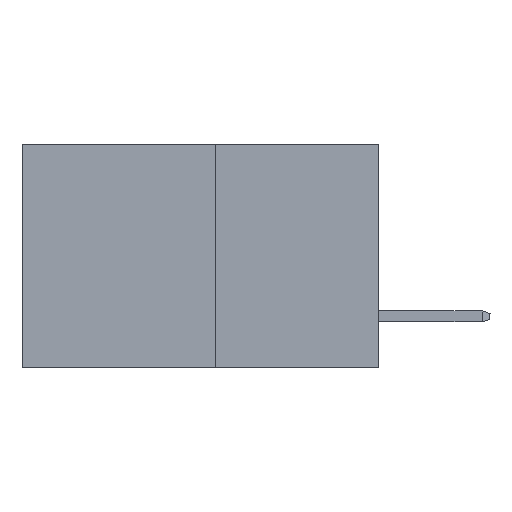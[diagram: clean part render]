
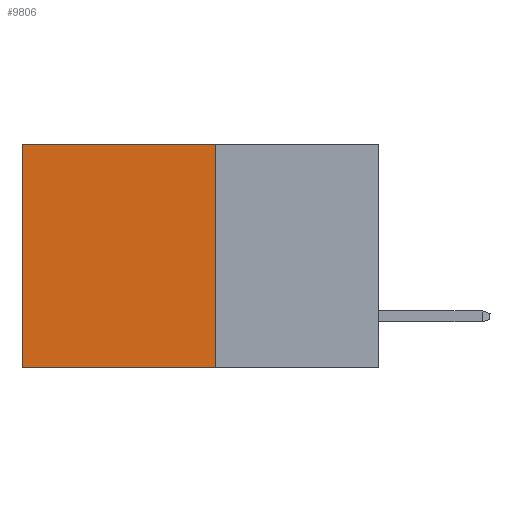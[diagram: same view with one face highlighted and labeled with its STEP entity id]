
A CAD part, left-side view. The second image highlights one B-rep face of the part: STEP entity #9806.
In plain terms, the highlighted planar face has unit normal (-1, 0, 0).
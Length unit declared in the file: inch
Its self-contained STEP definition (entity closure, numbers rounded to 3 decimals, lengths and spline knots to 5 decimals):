
#234 = DIRECTION ( 'NONE',  ( 0., 0., -1. ) ) ;
#895 = LINE ( 'NONE', #8457, #8799 ) ;
#994 = ORIENTED_EDGE ( 'NONE', *, *, #8426, .F. ) ;
#1019 = LINE ( 'NONE', #6784, #7159 ) ;
#1117 = CARTESIAN_POINT ( 'NONE',  ( 0.277, 0.27, -0.37 ) ) ;
#1281 = VERTEX_POINT ( 'NONE', #1923 ) ;
#1366 = VECTOR ( 'NONE', #7724, 39.37008 ) ;
#1373 = DIRECTION ( 'NONE',  ( 1., 0., 0. ) ) ;
#1496 = ORIENTED_EDGE ( 'NONE', *, *, #9750, .T. ) ;
#1528 = VECTOR ( 'NONE', #1953, 39.37008 ) ;
#1857 = VERTEX_POINT ( 'NONE', #4063 ) ;
#1923 = CARTESIAN_POINT ( 'NONE',  ( 0.277, 0.59, 0. ) ) ;
#1953 = DIRECTION ( 'NONE',  ( 0., 1., 0. ) ) ;
#2244 = CARTESIAN_POINT ( 'NONE',  ( 0.277, 0.59, -0.37 ) ) ;
#3518 = LINE ( 'NONE', #9113, #1366 ) ;
#3778 = VERTEX_POINT ( 'NONE', #9079 ) ;
#3937 = LINE ( 'NONE', #1117, #1528 ) ;
#4063 = CARTESIAN_POINT ( 'NONE',  ( 0.277, 0.27, -0.37 ) ) ;
#4882 = EDGE_CURVE ( 'NONE', #1281, #9872, #895, .T. ) ;
#5848 = ORIENTED_EDGE ( 'NONE', *, *, #4882, .T. ) ;
#6466 = EDGE_LOOP ( 'NONE', ( #5848, #8527, #994, #1496 ) ) ;
#6784 = CARTESIAN_POINT ( 'NONE',  ( 0.277, 0.27, -0.37 ) ) ;
#6917 = CARTESIAN_POINT ( 'NONE',  ( 0.277, 0.27, -0.37 ) ) ;
#6953 = DIRECTION ( 'NONE',  ( 0., 0., -1. ) ) ;
#7159 = VECTOR ( 'NONE', #7606, 39.37008 ) ;
#7515 = FACE_OUTER_BOUND ( 'NONE', #6466, .T. ) ;
#7606 = DIRECTION ( 'NONE',  ( 0., 0., -1. ) ) ;
#7724 = DIRECTION ( 'NONE',  ( 0., 1., 0. ) ) ;
#8370 = EDGE_CURVE ( 'NONE', #1857, #9872, #3937, .T. ) ;
#8426 = EDGE_CURVE ( 'NONE', #3778, #1857, #1019, .T. ) ;
#8457 = CARTESIAN_POINT ( 'NONE',  ( 0.277, 0.59, -0.37 ) ) ;
#8527 = ORIENTED_EDGE ( 'NONE', *, *, #8370, .F. ) ;
#8799 = VECTOR ( 'NONE', #234, 39.37008 ) ;
#9079 = CARTESIAN_POINT ( 'NONE',  ( 0.277, 0.27, 0. ) ) ;
#9113 = CARTESIAN_POINT ( 'NONE',  ( 0.277, 0.27, 0. ) ) ;
#9750 = EDGE_CURVE ( 'NONE', #3778, #1281, #3518, .T. ) ;
#9806 = ADVANCED_FACE ( 'NONE', ( #7515 ), #9904, .F. ) ;
#9872 = VERTEX_POINT ( 'NONE', #2244 ) ;
#9904 = PLANE ( 'NONE',  #9924 ) ;
#9924 = AXIS2_PLACEMENT_3D ( 'NONE', #6917, #1373, #6953 ) ;
